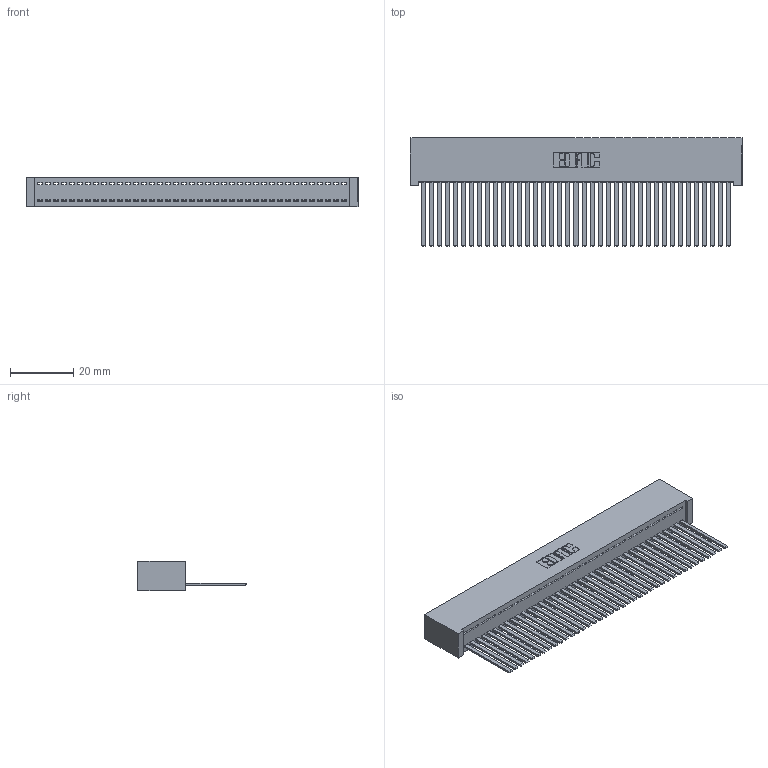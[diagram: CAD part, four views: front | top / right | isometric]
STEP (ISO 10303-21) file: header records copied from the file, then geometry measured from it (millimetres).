
FILE_DESCRIPTION (( 'STEP AP203' ), '1' );
FILE_NAME ('392-039-544-101.STEP', '2018-08-16T06:37:07', ( '' ), ( '' ), 'SwSTEP 2.0', 'SolidWorks 2016', '' );
FILE_SCHEMA (( 'CONFIG_CONTROL_DESIGN' ));
Length unit declared in the file: inch
Products named in the file (3): 392-039-544-101; 342 Part_Lugless; 345-292-001_345-293-144
Assembly tree (40 placements, depth 2):
  392-039-544-101
    342 Part_Lugless
    345-292-001_345-293-144  x39
Bounding box: 105.31 x 34.3 x 9.4 mm (x, y, z)
Volume: 10083 mm3; surface area: 16359.3 mm2
Topology: 40 solids, 40 shells, 2130 faces, 6437 edges, 4238 vertices
Faces by surface type: plane 1544, cylinder 586
Entity records: 23637 total; most frequent: CARTESIAN_POINT 4083, ORIENTED_EDGE 4058, DIRECTION 3439, EDGE_CURVE 2029, VECTOR 1913, LINE 1913, VERTEX_POINT 1350, AXIS2_PLACEMENT_3D 763
